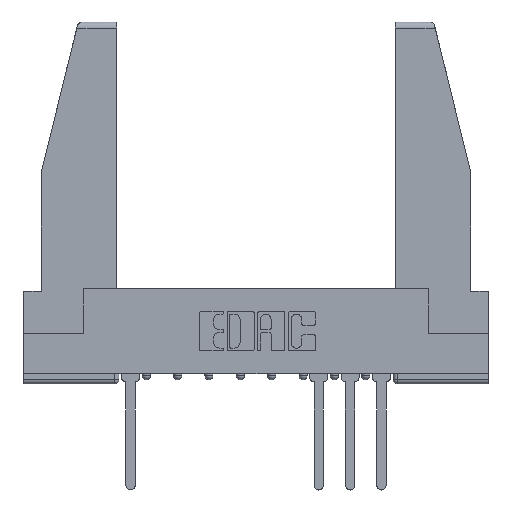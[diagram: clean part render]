
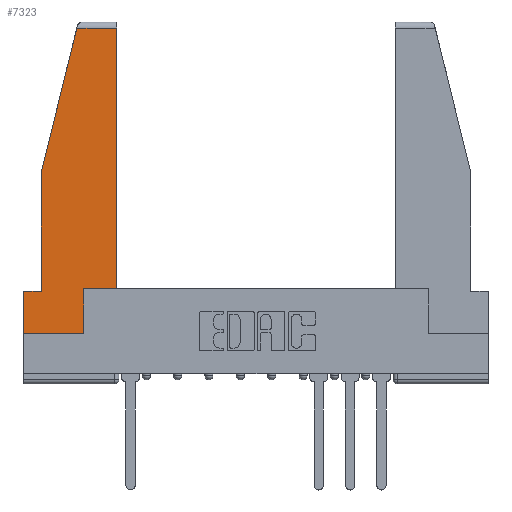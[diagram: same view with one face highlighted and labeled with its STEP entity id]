
A CAD part, top view. The second image highlights one B-rep face of the part: STEP entity #7323.
In plain terms, the highlighted planar face has unit normal (0, 0, 1).
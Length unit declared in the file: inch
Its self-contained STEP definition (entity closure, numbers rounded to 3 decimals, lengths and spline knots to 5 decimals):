
#52 = VECTOR ( 'NONE', #9722, 39.37008 ) ;
#122 = DIRECTION ( 'NONE',  ( 0., 0., 1. ) ) ;
#591 = CARTESIAN_POINT ( 'NONE',  ( 0.297, 0.223, 0. ) ) ;
#688 = VECTOR ( 'NONE', #4506, 39.37008 ) ;
#745 = CARTESIAN_POINT ( 'NONE',  ( 0.297, 0., 0. ) ) ;
#794 = EDGE_CURVE ( 'NONE', #12733, #5448, #7482, .T. ) ;
#1259 = VECTOR ( 'NONE', #5230, 39.37008 ) ;
#1418 = CARTESIAN_POINT ( 'NONE',  ( 0., 0., 0. ) ) ;
#1439 = CARTESIAN_POINT ( 'NONE',  ( 0.086, 0.8, 0. ) ) ;
#1839 = FACE_OUTER_BOUND ( 'NONE', #2977, .T. ) ;
#2011 = VECTOR ( 'NONE', #9458, 39.37008 ) ;
#2113 = CARTESIAN_POINT ( 'NONE',  ( 0.461, 1.52, 0. ) ) ;
#2161 = CARTESIAN_POINT ( 'NONE',  ( 0.271, 1.55, 0. ) ) ;
#2231 = VERTEX_POINT ( 'NONE', #6870 ) ;
#2313 = ORIENTED_EDGE ( 'NONE', *, *, #11170, .T. ) ;
#2655 = ORIENTED_EDGE ( 'NONE', *, *, #11722, .T. ) ;
#2977 = EDGE_LOOP ( 'NONE', ( #3110, #9300, #10012, #11019, #11803, #2313, #9745, #2655, #9083 ) ) ;
#3067 = DIRECTION ( 'NONE',  ( 0., -1., 0. ) ) ;
#3110 = ORIENTED_EDGE ( 'NONE', *, *, #9046, .T. ) ;
#3149 = EDGE_CURVE ( 'NONE', #7389, #2231, #7092, .T. ) ;
#3184 = LINE ( 'NONE', #8412, #8563 ) ;
#3276 = DIRECTION ( 'NONE',  ( -0.239, -0.971, 0. ) ) ;
#3411 = CARTESIAN_POINT ( 'NONE',  ( 0., 0.21, 0. ) ) ;
#3419 = VERTEX_POINT ( 'NONE', #1418 ) ;
#3552 = CARTESIAN_POINT ( 'NONE',  ( 0., 0., 0. ) ) ;
#4048 = LINE ( 'NONE', #5636, #688 ) ;
#4223 = VECTOR ( 'NONE', #6416, 39.37008 ) ;
#4506 = DIRECTION ( 'NONE',  ( 0., 1., 0. ) ) ;
#5230 = DIRECTION ( 'NONE',  ( -1., 0., 0. ) ) ;
#5244 = DIRECTION ( 'NONE',  ( 1., 0., 0. ) ) ;
#5448 = VERTEX_POINT ( 'NONE', #7686 ) ;
#5636 = CARTESIAN_POINT ( 'NONE',  ( 0.461, 0.223, 0. ) ) ;
#6037 = EDGE_CURVE ( 'NONE', #3419, #11431, #12750, .T. ) ;
#6414 = CARTESIAN_POINT ( 'NONE',  ( 0.086, 0.8, 0. ) ) ;
#6416 = DIRECTION ( 'NONE',  ( 0., -1., 0. ) ) ;
#6602 = LINE ( 'NONE', #745, #12501 ) ;
#6791 = CARTESIAN_POINT ( 'NONE',  ( 0.297, 0., 0. ) ) ;
#6864 = PLANE ( 'NONE',  #11331 ) ;
#6870 = CARTESIAN_POINT ( 'NONE',  ( 0.086, 0.21, 0. ) ) ;
#7092 = LINE ( 'NONE', #6414, #4223 ) ;
#7323 = ADVANCED_FACE ( 'NONE', ( #1839 ), #6864, .T. ) ;
#7389 = VERTEX_POINT ( 'NONE', #1439 ) ;
#7482 = LINE ( 'NONE', #11001, #2011 ) ;
#7686 = CARTESIAN_POINT ( 'NONE',  ( 0.461, 0.223, 0. ) ) ;
#7846 = VERTEX_POINT ( 'NONE', #12071 ) ;
#7891 = DIRECTION ( 'NONE',  ( 1., 0., 0. ) ) ;
#8191 = LINE ( 'NONE', #13882, #52 ) ;
#8397 = DIRECTION ( 'NONE',  ( 0., 1., 0. ) ) ;
#8412 = CARTESIAN_POINT ( 'NONE',  ( 0., 0.21, 0. ) ) ;
#8563 = VECTOR ( 'NONE', #3067, 39.37008 ) ;
#8703 = CARTESIAN_POINT ( 'NONE',  ( 0., 0., 0. ) ) ;
#8773 = EDGE_CURVE ( 'NONE', #10152, #7846, #9923, .T. ) ;
#8931 = EDGE_CURVE ( 'NONE', #7846, #7389, #10395, .T. ) ;
#9046 = EDGE_CURVE ( 'NONE', #5448, #10152, #4048, .T. ) ;
#9083 = ORIENTED_EDGE ( 'NONE', *, *, #794, .T. ) ;
#9300 = ORIENTED_EDGE ( 'NONE', *, *, #8773, .T. ) ;
#9458 = DIRECTION ( 'NONE',  ( 1., 0., 0. ) ) ;
#9722 = DIRECTION ( 'NONE',  ( -1., 0., 0. ) ) ;
#9745 = ORIENTED_EDGE ( 'NONE', *, *, #6037, .T. ) ;
#9923 = LINE ( 'NONE', #11531, #1259 ) ;
#10012 = ORIENTED_EDGE ( 'NONE', *, *, #8931, .T. ) ;
#10152 = VERTEX_POINT ( 'NONE', #2113 ) ;
#10395 = LINE ( 'NONE', #2161, #13500 ) ;
#11001 = CARTESIAN_POINT ( 'NONE',  ( 0.297, 0.223, 0. ) ) ;
#11019 = ORIENTED_EDGE ( 'NONE', *, *, #3149, .T. ) ;
#11170 = EDGE_CURVE ( 'NONE', #11937, #3419, #3184, .T. ) ;
#11331 = AXIS2_PLACEMENT_3D ( 'NONE', #3552, #122, #7891 ) ;
#11431 = VERTEX_POINT ( 'NONE', #6791 ) ;
#11531 = CARTESIAN_POINT ( 'NONE',  ( 0., 1.52, 0. ) ) ;
#11722 = EDGE_CURVE ( 'NONE', #11431, #12733, #6602, .T. ) ;
#11803 = ORIENTED_EDGE ( 'NONE', *, *, #12935, .T. ) ;
#11937 = VERTEX_POINT ( 'NONE', #3411 ) ;
#12071 = CARTESIAN_POINT ( 'NONE',  ( 0.2636, 1.52, 0. ) ) ;
#12431 = VECTOR ( 'NONE', #5244, 39.37008 ) ;
#12501 = VECTOR ( 'NONE', #8397, 39.37008 ) ;
#12733 = VERTEX_POINT ( 'NONE', #591 ) ;
#12750 = LINE ( 'NONE', #8703, #12431 ) ;
#12935 = EDGE_CURVE ( 'NONE', #2231, #11937, #8191, .T. ) ;
#13500 = VECTOR ( 'NONE', #3276, 39.37008 ) ;
#13882 = CARTESIAN_POINT ( 'NONE',  ( 0., 0.21, 0. ) ) ;
